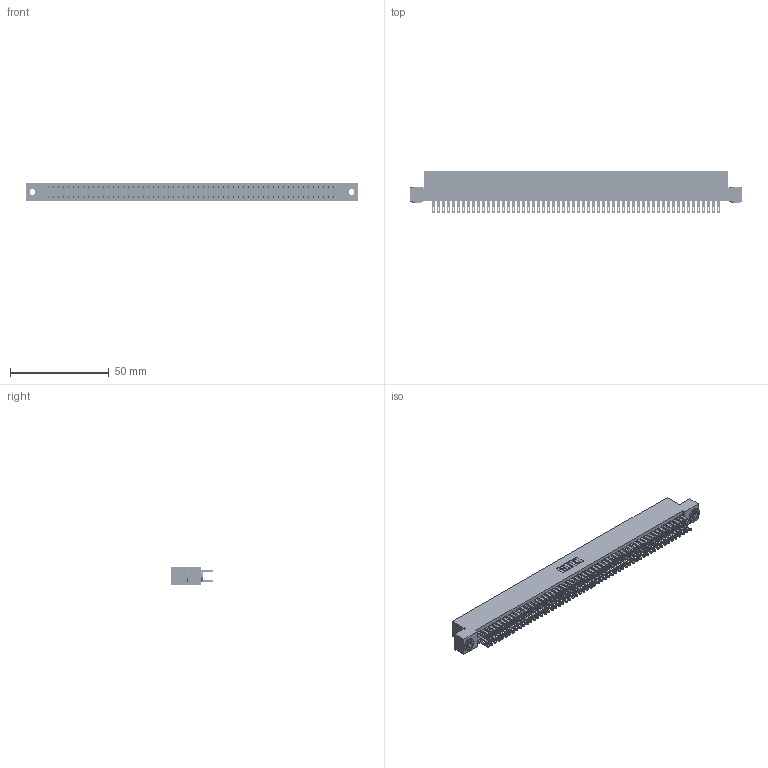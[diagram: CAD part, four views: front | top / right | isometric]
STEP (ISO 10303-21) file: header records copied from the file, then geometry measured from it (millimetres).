
FILE_DESCRIPTION (( 'STEP AP203' ), '1' );
FILE_NAME ('345-116-500-203.STEP', '2019-11-05T13:30:46', ( '' ), ( '' ), 'SwSTEP 2.0', 'SolidWorks 2016', '' );
FILE_SCHEMA (( 'CONFIG_CONTROL_DESIGN' ));
Length unit declared in the file: inch
Products named in the file (4): 345-292-001_345-293-100; 345-116-500-203; 345-250-002_345-250-002-102; 345 Part_Flush Mounting Lugs - 0.156 Dia-TH
Assembly tree (119 placements, depth 2):
  345-116-500-203
    345 Part_Flush Mounting Lugs - 0.156 Dia-TH
    345-292-001_345-293-100  x116
    345-250-002_345-250-002-102  x2
Bounding box: 168.53 x 21.51 x 9.4 mm (x, y, z)
Volume: 16893.5 mm3; surface area: 26669.3 mm2
Topology: 119 solids, 119 shells, 5500 faces, 16773 edges, 11178 vertices
Faces by surface type: plane 3222, cylinder 2270, cone 8
Entity records: 43934 total; most frequent: CARTESIAN_POINT 7323, ORIENTED_EDGE 7250, DIRECTION 6471, EDGE_CURVE 3625, LINE 3233, VECTOR 3233, VERTEX_POINT 2414, AXIS2_PLACEMENT_3D 1619
